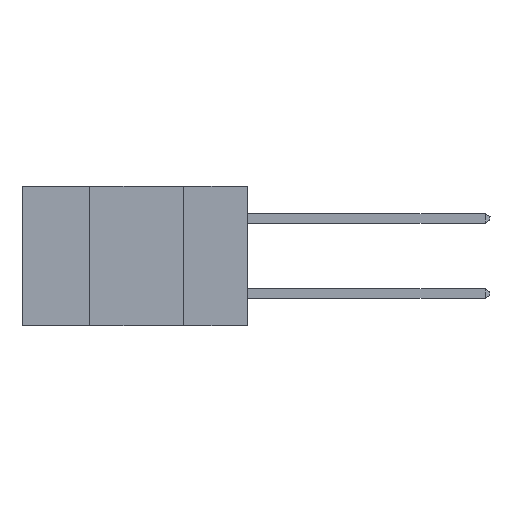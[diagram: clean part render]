
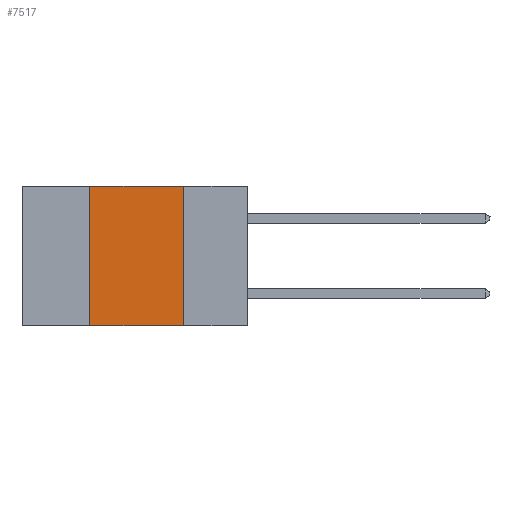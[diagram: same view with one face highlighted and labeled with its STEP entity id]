
A CAD part, left-side view. The second image highlights one B-rep face of the part: STEP entity #7517.
In plain terms, the highlighted planar face has unit normal (-1, 0, 0).
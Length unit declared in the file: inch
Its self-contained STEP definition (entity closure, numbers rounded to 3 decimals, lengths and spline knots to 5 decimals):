
#557 = CARTESIAN_POINT ( 'NONE',  ( 0., 0.17, 0. ) ) ;
#738 = ORIENTED_EDGE ( 'NONE', *, *, #19198, .F. ) ;
#2845 = ORIENTED_EDGE ( 'NONE', *, *, #7836, .F. ) ;
#3131 = DIRECTION ( 'NONE',  ( 0., -1., 0. ) ) ;
#3151 = AXIS2_PLACEMENT_3D ( 'NONE', #23564, #21557, #11565 ) ;
#3431 = VERTEX_POINT ( 'NONE', #4408 ) ;
#3448 = PLANE ( 'NONE',  #3151 ) ;
#3999 = LINE ( 'NONE', #12095, #16041 ) ;
#4408 = CARTESIAN_POINT ( 'NONE',  ( 0., 0.42, 0. ) ) ;
#4429 = EDGE_CURVE ( 'NONE', #16721, #20831, #14645, .T. ) ;
#4526 = CARTESIAN_POINT ( 'NONE',  ( 0., 0.17, -0.37 ) ) ;
#5165 = EDGE_LOOP ( 'NONE', ( #21076, #2845, #738, #19227 ) ) ;
#5377 = CARTESIAN_POINT ( 'NONE',  ( 0., 0.42, -0.37 ) ) ;
#7517 = ADVANCED_FACE ( 'NONE', ( #12035 ), #3448, .F. ) ;
#7769 = DIRECTION ( 'NONE',  ( 0., 0., 1. ) ) ;
#7836 = EDGE_CURVE ( 'NONE', #3431, #16721, #19252, .T. ) ;
#10301 = VECTOR ( 'NONE', #7769, 39.37008 ) ;
#10961 = CARTESIAN_POINT ( 'NONE',  ( 0., 0.17, -0.37 ) ) ;
#11510 = LINE ( 'NONE', #5377, #10301 ) ;
#11565 = DIRECTION ( 'NONE',  ( 0., 0., -1. ) ) ;
#11903 = CARTESIAN_POINT ( 'NONE',  ( 0., 0.42, -0.37 ) ) ;
#12035 = FACE_OUTER_BOUND ( 'NONE', #5165, .T. ) ;
#12095 = CARTESIAN_POINT ( 'NONE',  ( 0., 0.6, -0.37 ) ) ;
#12630 = DIRECTION ( 'NONE',  ( 0., 0., -1. ) ) ;
#12875 = VERTEX_POINT ( 'NONE', #11903 ) ;
#14247 = DIRECTION ( 'NONE',  ( 0., -1., 0. ) ) ;
#14645 = LINE ( 'NONE', #4526, #17622 ) ;
#15384 = CARTESIAN_POINT ( 'NONE',  ( 0., 0.6, 0. ) ) ;
#16041 = VECTOR ( 'NONE', #14247, 39.37008 ) ;
#16721 = VERTEX_POINT ( 'NONE', #557 ) ;
#17622 = VECTOR ( 'NONE', #12630, 39.37008 ) ;
#19198 = EDGE_CURVE ( 'NONE', #12875, #3431, #11510, .T. ) ;
#19227 = ORIENTED_EDGE ( 'NONE', *, *, #24405, .T. ) ;
#19252 = LINE ( 'NONE', #15384, #21426 ) ;
#20831 = VERTEX_POINT ( 'NONE', #10961 ) ;
#21076 = ORIENTED_EDGE ( 'NONE', *, *, #4429, .F. ) ;
#21426 = VECTOR ( 'NONE', #3131, 39.37008 ) ;
#21557 = DIRECTION ( 'NONE',  ( 1., 0., 0. ) ) ;
#23564 = CARTESIAN_POINT ( 'NONE',  ( 0., 0.6, 0. ) ) ;
#24405 = EDGE_CURVE ( 'NONE', #12875, #20831, #3999, .T. ) ;
